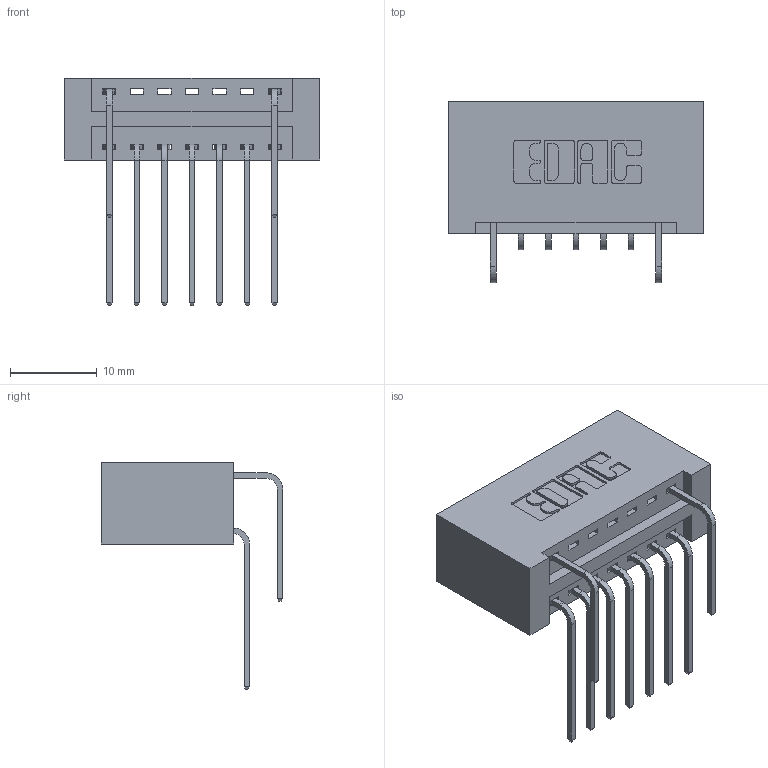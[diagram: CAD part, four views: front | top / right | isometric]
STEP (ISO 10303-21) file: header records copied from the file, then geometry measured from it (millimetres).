
FILE_DESCRIPTION (( 'STEP AP203' ), '1' );
FILE_NAME ('346-014-559-201.STEP', '2018-08-20T02:01:20', ( '' ), ( '' ), 'SwSTEP 2.0', 'SolidWorks 2016', '' );
FILE_SCHEMA (( 'CONFIG_CONTROL_DESIGN' ));
Length unit declared in the file: inch
Products named in the file (4): 346 Part_No Mounting Lugs; 345-292-001_558 559 Tail - 1; 345-292-001_559 Tail - 2; 346-014-559-201
Assembly tree (10 placements, depth 2):
  346-014-559-201
    346 Part_No Mounting Lugs
    345-292-001_558 559 Tail - 1  x7
    345-292-001_559 Tail - 2  x2
Bounding box: 29.46 x 20.89 x 26.16 mm (x, y, z)
Volume: 3181.5 mm3; surface area: 3975.8 mm2
Topology: 10 solids, 10 shells, 630 faces, 1859 edges, 1226 vertices
Faces by surface type: plane 430, cylinder 200
Entity records: 10627 total; most frequent: CARTESIAN_POINT 1870, ORIENTED_EDGE 1758, DIRECTION 1661, EDGE_CURVE 879, VECTOR 687, LINE 687, VERTEX_POINT 582, AXIS2_PLACEMENT_3D 487
